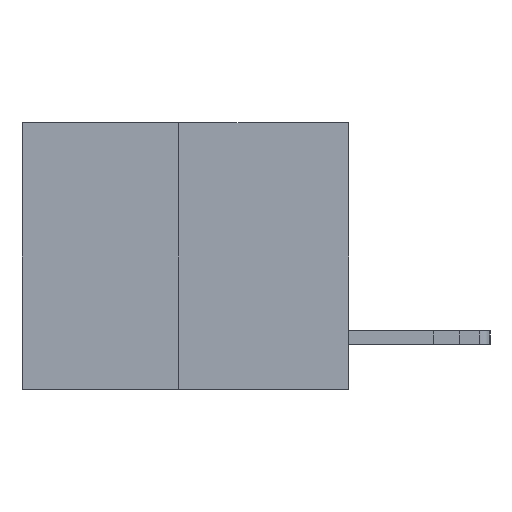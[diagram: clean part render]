
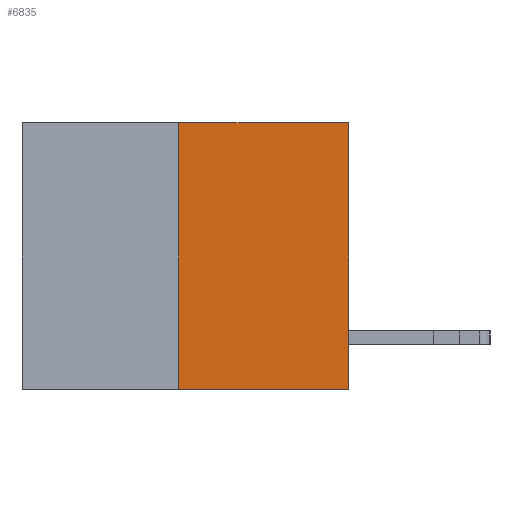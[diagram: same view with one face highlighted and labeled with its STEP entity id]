
A CAD part, left-side view. The second image highlights one B-rep face of the part: STEP entity #6835.
In plain terms, the highlighted planar face has unit normal (-1, 0, 0).
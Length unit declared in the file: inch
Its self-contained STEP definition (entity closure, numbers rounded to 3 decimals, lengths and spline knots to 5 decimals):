
#484 = DIRECTION ( 'NONE',  ( 0., 0., -1. ) ) ;
#672 = CARTESIAN_POINT ( 'NONE',  ( 0., 0.312, 0. ) ) ;
#940 = DIRECTION ( 'NONE',  ( 0., 0., 1. ) ) ;
#959 = LINE ( 'NONE', #14960, #10419 ) ;
#1239 = CARTESIAN_POINT ( 'NONE',  ( 0., 0., 0. ) ) ;
#1386 = VERTEX_POINT ( 'NONE', #672 ) ;
#3966 = CARTESIAN_POINT ( 'NONE',  ( 0., 0.312, -0.49 ) ) ;
#4416 = LINE ( 'NONE', #10839, #12677 ) ;
#5240 = PLANE ( 'NONE',  #14201 ) ;
#5414 = CARTESIAN_POINT ( 'NONE',  ( 0., 0., -0.49 ) ) ;
#6080 = EDGE_CURVE ( 'NONE', #7308, #13480, #16407, .T. ) ;
#6270 = EDGE_LOOP ( 'NONE', ( #9216, #15898, #15036, #10058 ) ) ;
#6835 = ADVANCED_FACE ( 'NONE', ( #7379 ), #5240, .F. ) ;
#7308 = VERTEX_POINT ( 'NONE', #5414 ) ;
#7379 = FACE_OUTER_BOUND ( 'NONE', #6270, .T. ) ;
#7728 = VECTOR ( 'NONE', #11605, 39.37008 ) ;
#7888 = CARTESIAN_POINT ( 'NONE',  ( 0., 0.6, 0. ) ) ;
#9050 = DIRECTION ( 'NONE',  ( 0., -1., 0. ) ) ;
#9216 = ORIENTED_EDGE ( 'NONE', *, *, #11630, .F. ) ;
#9605 = CARTESIAN_POINT ( 'NONE',  ( 0., 0., 0. ) ) ;
#10058 = ORIENTED_EDGE ( 'NONE', *, *, #14258, .F. ) ;
#10419 = VECTOR ( 'NONE', #940, 39.37008 ) ;
#10839 = CARTESIAN_POINT ( 'NONE',  ( 0., 0.6, -0.49 ) ) ;
#11605 = DIRECTION ( 'NONE',  ( 0., 0., 1. ) ) ;
#11630 = EDGE_CURVE ( 'NONE', #12712, #1386, #959, .T. ) ;
#11991 = DIRECTION ( 'NONE',  ( 1., 0., 0. ) ) ;
#12677 = VECTOR ( 'NONE', #14931, 39.37008 ) ;
#12712 = VERTEX_POINT ( 'NONE', #3966 ) ;
#13148 = VECTOR ( 'NONE', #9050, 39.37008 ) ;
#13480 = VERTEX_POINT ( 'NONE', #9605 ) ;
#14201 = AXIS2_PLACEMENT_3D ( 'NONE', #15788, #11991, #484 ) ;
#14258 = EDGE_CURVE ( 'NONE', #1386, #13480, #14538, .T. ) ;
#14538 = LINE ( 'NONE', #7888, #13148 ) ;
#14931 = DIRECTION ( 'NONE',  ( 0., -1., 0. ) ) ;
#14960 = CARTESIAN_POINT ( 'NONE',  ( 0., 0.312, -0.49 ) ) ;
#15036 = ORIENTED_EDGE ( 'NONE', *, *, #6080, .T. ) ;
#15788 = CARTESIAN_POINT ( 'NONE',  ( 0., 0.6, 0. ) ) ;
#15898 = ORIENTED_EDGE ( 'NONE', *, *, #16392, .T. ) ;
#16392 = EDGE_CURVE ( 'NONE', #12712, #7308, #4416, .T. ) ;
#16407 = LINE ( 'NONE', #1239, #7728 ) ;
